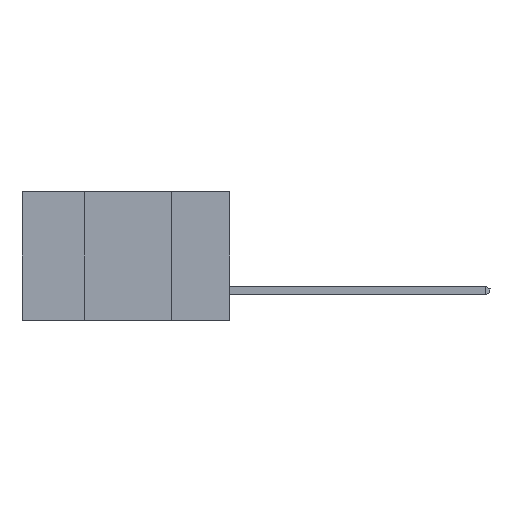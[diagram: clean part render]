
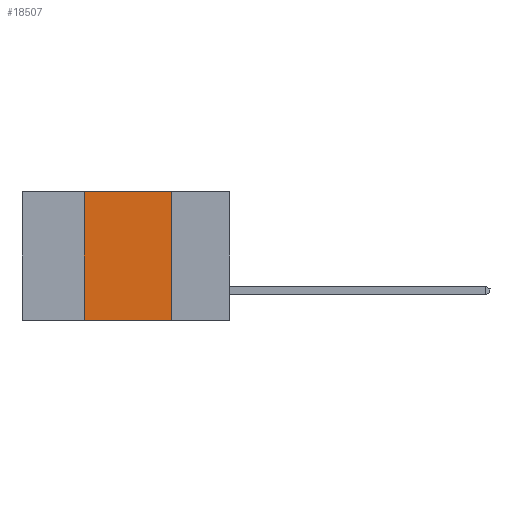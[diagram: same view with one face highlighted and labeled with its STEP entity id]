
A CAD part, left-side view. The second image highlights one B-rep face of the part: STEP entity #18507.
In plain terms, the highlighted planar face has unit normal (-1, 0, 0).
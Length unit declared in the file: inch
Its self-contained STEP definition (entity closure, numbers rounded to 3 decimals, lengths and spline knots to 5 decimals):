
#62 = EDGE_CURVE ( 'NONE', #8201, #10280, #18962, .T. ) ;
#416 = VECTOR ( 'NONE', #15020, 39.37008 ) ;
#715 = ORIENTED_EDGE ( 'NONE', *, *, #2720, .F. ) ;
#1259 = CARTESIAN_POINT ( 'NONE',  ( 0., 0.17, 0. ) ) ;
#1751 = LINE ( 'NONE', #18290, #416 ) ;
#1930 = EDGE_CURVE ( 'NONE', #8201, #17126, #17609, .T. ) ;
#2467 = DIRECTION ( 'NONE',  ( 1., 0., 0. ) ) ;
#2484 = DIRECTION ( 'NONE',  ( 0., -1., 0. ) ) ;
#2720 = EDGE_CURVE ( 'NONE', #8531, #17126, #1751, .T. ) ;
#3729 = CARTESIAN_POINT ( 'NONE',  ( 0., 0.42, -0.37 ) ) ;
#4206 = PLANE ( 'NONE',  #16555 ) ;
#5298 = CARTESIAN_POINT ( 'NONE',  ( 0., 0.17, -0.37 ) ) ;
#5704 = ORIENTED_EDGE ( 'NONE', *, *, #1930, .T. ) ;
#6765 = VECTOR ( 'NONE', #2484, 39.37008 ) ;
#7888 = CARTESIAN_POINT ( 'NONE',  ( 0., 0.42, 0. ) ) ;
#8201 = VERTEX_POINT ( 'NONE', #21209 ) ;
#8531 = VERTEX_POINT ( 'NONE', #1259 ) ;
#8844 = DIRECTION ( 'NONE',  ( 0., 0., 1. ) ) ;
#9242 = EDGE_CURVE ( 'NONE', #10280, #8531, #14120, .T. ) ;
#9299 = VECTOR ( 'NONE', #21003, 39.37008 ) ;
#10280 = VERTEX_POINT ( 'NONE', #7888 ) ;
#10626 = DIRECTION ( 'NONE',  ( 0., 0., -1. ) ) ;
#11187 = CARTESIAN_POINT ( 'NONE',  ( 0., 0.6, -0.37 ) ) ;
#11992 = CARTESIAN_POINT ( 'NONE',  ( 0., 0.6, 0. ) ) ;
#12155 = CARTESIAN_POINT ( 'NONE',  ( 0., 0.6, 0. ) ) ;
#13896 = ORIENTED_EDGE ( 'NONE', *, *, #9242, .F. ) ;
#14120 = LINE ( 'NONE', #11992, #6765 ) ;
#15020 = DIRECTION ( 'NONE',  ( 0., 0., -1. ) ) ;
#15798 = EDGE_LOOP ( 'NONE', ( #715, #13896, #21197, #5704 ) ) ;
#16555 = AXIS2_PLACEMENT_3D ( 'NONE', #12155, #2467, #10626 ) ;
#16635 = VECTOR ( 'NONE', #8844, 39.37008 ) ;
#17126 = VERTEX_POINT ( 'NONE', #5298 ) ;
#17476 = FACE_OUTER_BOUND ( 'NONE', #15798, .T. ) ;
#17609 = LINE ( 'NONE', #11187, #9299 ) ;
#18290 = CARTESIAN_POINT ( 'NONE',  ( 0., 0.17, -0.37 ) ) ;
#18507 = ADVANCED_FACE ( 'NONE', ( #17476 ), #4206, .F. ) ;
#18962 = LINE ( 'NONE', #3729, #16635 ) ;
#21003 = DIRECTION ( 'NONE',  ( 0., -1., 0. ) ) ;
#21197 = ORIENTED_EDGE ( 'NONE', *, *, #62, .F. ) ;
#21209 = CARTESIAN_POINT ( 'NONE',  ( 0., 0.42, -0.37 ) ) ;
